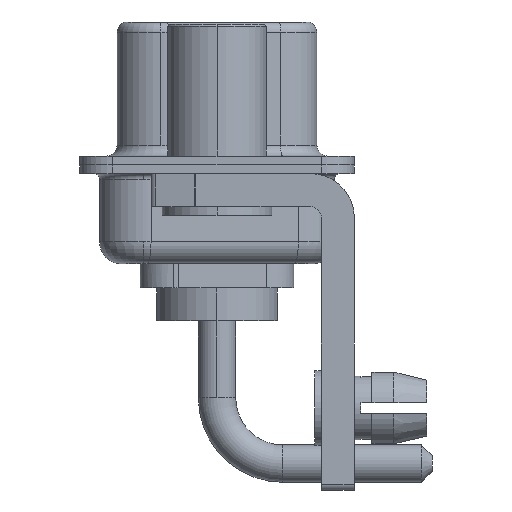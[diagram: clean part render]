
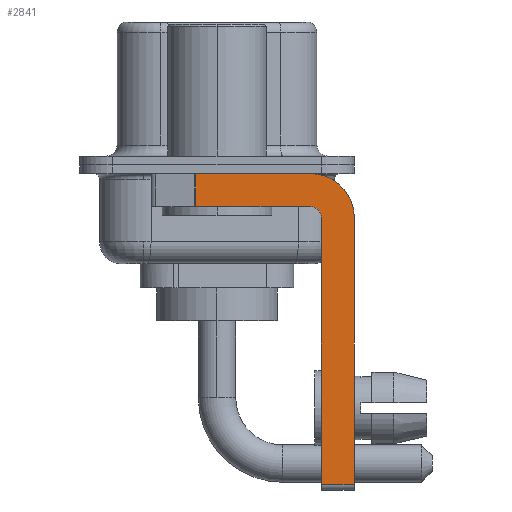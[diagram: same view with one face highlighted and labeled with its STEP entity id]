
A CAD part, left-side view. The second image highlights one B-rep face of the part: STEP entity #2841.
In plain terms, the highlighted planar face has unit normal (-1, 0, 0).
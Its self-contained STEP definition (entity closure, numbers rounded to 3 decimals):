
#138 = ORIENTED_EDGE ( 'NONE', *, *, #11888, .T. ) ;
#249 = LINE ( 'NONE', #9176, #8963 ) ;
#925 = DIRECTION ( 'NONE',  ( 0., -1., 0. ) ) ;
#1312 = CARTESIAN_POINT ( 'NONE',  ( -2.9, -4.25, -0.4 ) ) ;
#1479 = VERTEX_POINT ( 'NONE', #3974 ) ;
#1891 = ORIENTED_EDGE ( 'NONE', *, *, #14005, .F. ) ;
#2206 = CARTESIAN_POINT ( 'NONE',  ( -2.9, -4.25, -1.9 ) ) ;
#2527 = ORIENTED_EDGE ( 'NONE', *, *, #12733, .T. ) ;
#2790 = DIRECTION ( 'NONE',  ( -1., 0., 0. ) ) ;
#2841 = ADVANCED_FACE ( 'NONE', ( #8712 ), #17638, .F. ) ;
#3249 = ORIENTED_EDGE ( 'NONE', *, *, #16455, .F. ) ;
#3700 = EDGE_CURVE ( 'NONE', #9904, #15055, #10039, .T. ) ;
#3890 = DIRECTION ( 'NONE',  ( 0., 0., -1. ) ) ;
#3974 = CARTESIAN_POINT ( 'NONE',  ( -2.9, 0.978, -1.9 ) ) ;
#3978 = ORIENTED_EDGE ( 'NONE', *, *, #7626, .F. ) ;
#4045 = AXIS2_PLACEMENT_3D ( 'NONE', #13130, #2790, #19453 ) ;
#4146 = VERTEX_POINT ( 'NONE', #14134 ) ;
#4216 = ORIENTED_EDGE ( 'NONE', *, *, #9345, .F. ) ;
#4374 = CARTESIAN_POINT ( 'NONE',  ( -2.9, 0.978, -0.4 ) ) ;
#4770 = VERTEX_POINT ( 'NONE', #6946 ) ;
#6343 = DIRECTION ( 'NONE',  ( 0., -1., 0. ) ) ;
#6575 = DIRECTION ( 'NONE',  ( 0., 0., -1. ) ) ;
#6946 = CARTESIAN_POINT ( 'NONE',  ( -2.9, -4.75, -2.4 ) ) ;
#7045 = CIRCLE ( 'NONE', #13777, 2. ) ;
#7192 = VERTEX_POINT ( 'NONE', #14847 ) ;
#7526 = EDGE_CURVE ( 'NONE', #19541, #1479, #8413, .T. ) ;
#7626 = EDGE_CURVE ( 'NONE', #16723, #4146, #11632, .T. ) ;
#8193 = VECTOR ( 'NONE', #19558, 1000. ) ;
#8413 = LINE ( 'NONE', #13322, #17483 ) ;
#8512 = CARTESIAN_POINT ( 'NONE',  ( -2.9, -6.25, -2.4 ) ) ;
#8712 = FACE_OUTER_BOUND ( 'NONE', #15058, .T. ) ;
#8730 = DIRECTION ( 'NONE',  ( 0., 0., -1. ) ) ;
#8866 = CIRCLE ( 'NONE', #4045, 0.5 ) ;
#8963 = VECTOR ( 'NONE', #6343, 1000. ) ;
#9176 = CARTESIAN_POINT ( 'NONE',  ( -2.9, -4.25, -14.55 ) ) ;
#9302 = LINE ( 'NONE', #17113, #16675 ) ;
#9345 = EDGE_CURVE ( 'NONE', #7192, #4770, #19426, .T. ) ;
#9856 = VECTOR ( 'NONE', #16399, 1000. ) ;
#9904 = VERTEX_POINT ( 'NONE', #4374 ) ;
#10039 = LINE ( 'NONE', #10136, #12926 ) ;
#10136 = CARTESIAN_POINT ( 'NONE',  ( -2.9, 3., -0.4 ) ) ;
#10212 = CARTESIAN_POINT ( 'NONE',  ( -2.9, -4.25, -2.4 ) ) ;
#11632 = LINE ( 'NONE', #8512, #8193 ) ;
#11732 = DIRECTION ( 'NONE',  ( 1., 0., 0. ) ) ;
#11888 = EDGE_CURVE ( 'NONE', #7192, #4146, #249, .T. ) ;
#12694 = CARTESIAN_POINT ( 'NONE',  ( -2.9, -6.25, -2.4 ) ) ;
#12733 = EDGE_CURVE ( 'NONE', #9904, #1479, #9302, .T. ) ;
#12926 = VECTOR ( 'NONE', #925, 1000. ) ;
#13130 = CARTESIAN_POINT ( 'NONE',  ( -2.9, -4.25, -2.4 ) ) ;
#13322 = CARTESIAN_POINT ( 'NONE',  ( -2.9, -4.25, -1.9 ) ) ;
#13530 = DIRECTION ( 'NONE',  ( 0., 1., 0. ) ) ;
#13613 = AXIS2_PLACEMENT_3D ( 'NONE', #10212, #16319, #3890 ) ;
#13777 = AXIS2_PLACEMENT_3D ( 'NONE', #19371, #11732, #8730 ) ;
#14005 = EDGE_CURVE ( 'NONE', #15055, #16723, #7045, .T. ) ;
#14134 = CARTESIAN_POINT ( 'NONE',  ( -2.9, -6.25, -14.55 ) ) ;
#14847 = CARTESIAN_POINT ( 'NONE',  ( -2.9, -4.75, -14.55 ) ) ;
#15055 = VERTEX_POINT ( 'NONE', #1312 ) ;
#15058 = EDGE_LOOP ( 'NONE', ( #19259, #2527, #19172, #3249, #4216, #138, #3978, #1891 ) ) ;
#16319 = DIRECTION ( 'NONE',  ( 1., 0., 0. ) ) ;
#16399 = DIRECTION ( 'NONE',  ( 0., 0., 1. ) ) ;
#16455 = EDGE_CURVE ( 'NONE', #4770, #19541, #8866, .T. ) ;
#16675 = VECTOR ( 'NONE', #6575, 1000. ) ;
#16723 = VERTEX_POINT ( 'NONE', #12694 ) ;
#17113 = CARTESIAN_POINT ( 'NONE',  ( -2.9, 0.978, -1.9 ) ) ;
#17483 = VECTOR ( 'NONE', #13530, 1000. ) ;
#17638 = PLANE ( 'NONE',  #13613 ) ;
#18110 = CARTESIAN_POINT ( 'NONE',  ( -2.9, -4.75, -14.8 ) ) ;
#19172 = ORIENTED_EDGE ( 'NONE', *, *, #7526, .F. ) ;
#19259 = ORIENTED_EDGE ( 'NONE', *, *, #3700, .F. ) ;
#19371 = CARTESIAN_POINT ( 'NONE',  ( -2.9, -4.25, -2.4 ) ) ;
#19426 = LINE ( 'NONE', #18110, #9856 ) ;
#19453 = DIRECTION ( 'NONE',  ( 0., 0., 1. ) ) ;
#19541 = VERTEX_POINT ( 'NONE', #2206 ) ;
#19558 = DIRECTION ( 'NONE',  ( 0., 0., -1. ) ) ;
